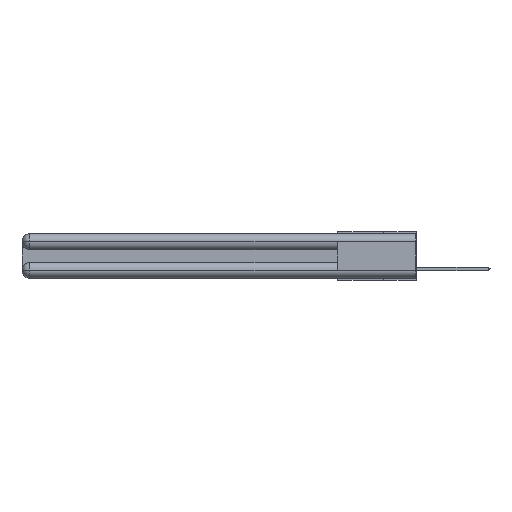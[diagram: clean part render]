
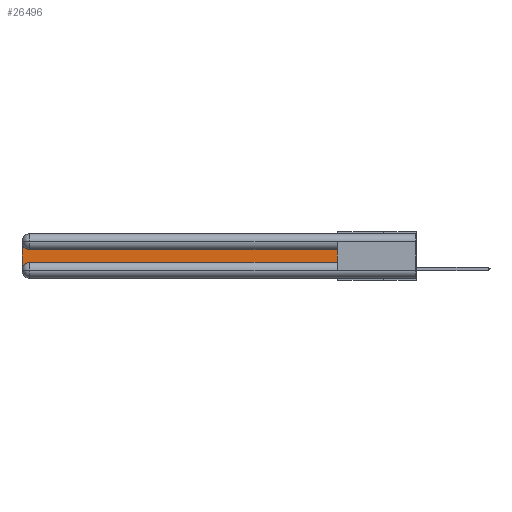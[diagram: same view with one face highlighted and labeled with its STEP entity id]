
A CAD part, left-side view. The second image highlights one B-rep face of the part: STEP entity #26496.
In plain terms, the highlighted planar face has unit normal (-1, 0, 0).
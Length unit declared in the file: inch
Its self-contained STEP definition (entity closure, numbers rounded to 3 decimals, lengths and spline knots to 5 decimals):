
#436 = CARTESIAN_POINT ( 'NONE',  ( 0.075, 2.94, -0.0625 ) ) ;
#612 = ORIENTED_EDGE ( 'NONE', *, *, #9793, .T. ) ;
#1330 = CARTESIAN_POINT ( 'NONE',  ( 0.075, 2.94, -0.2175 ) ) ;
#1367 = CARTESIAN_POINT ( 'NONE',  ( 0.075, 0.6, -0.2175 ) ) ;
#1648 = VERTEX_POINT ( 'NONE', #19882 ) ;
#1867 = DIRECTION ( 'NONE',  ( 0., 0., -1. ) ) ;
#1879 = DIRECTION ( 'NONE',  ( 0., 1., 0. ) ) ;
#2071 = ORIENTED_EDGE ( 'NONE', *, *, #19407, .T. ) ;
#2129 = PLANE ( 'NONE',  #17156 ) ;
#2230 = LINE ( 'NONE', #1367, #27242 ) ;
#2423 = EDGE_LOOP ( 'NONE', ( #29023, #2071, #612, #17621, #30944, #19347 ) ) ;
#3076 = VERTEX_POINT ( 'NONE', #3538 ) ;
#3538 = CARTESIAN_POINT ( 'NONE',  ( 0.075, 2.94, -0.1225 ) ) ;
#5513 = FACE_OUTER_BOUND ( 'NONE', #2423, .T. ) ;
#5653 = DIRECTION ( 'NONE',  ( 1., 0., 0. ) ) ;
#6305 = CARTESIAN_POINT ( 'NONE',  ( 0.075, 3., -0.0625 ) ) ;
#6504 = AXIS2_PLACEMENT_3D ( 'NONE', #436, #5653, #7780 ) ;
#7027 = DIRECTION ( 'NONE',  ( 0., 0., -1. ) ) ;
#7780 = DIRECTION ( 'NONE',  ( 0., 0., -1. ) ) ;
#8475 = VECTOR ( 'NONE', #19235, 39.37008 ) ;
#8689 = VERTEX_POINT ( 'NONE', #6305 ) ;
#9124 = DIRECTION ( 'NONE',  ( 1., 0., 0. ) ) ;
#9793 = EDGE_CURVE ( 'NONE', #8689, #20621, #13392, .T. ) ;
#11976 = CARTESIAN_POINT ( 'NONE',  ( 0.075, 3., -0.1225 ) ) ;
#13082 = CIRCLE ( 'NONE', #6504, 0.06 ) ;
#13392 = LINE ( 'NONE', #21542, #8475 ) ;
#15097 = DIRECTION ( 'NONE',  ( 0., 0., 1. ) ) ;
#15887 = VECTOR ( 'NONE', #15097, 39.37008 ) ;
#16566 = EDGE_CURVE ( 'NONE', #18988, #1648, #20831, .T. ) ;
#17156 = AXIS2_PLACEMENT_3D ( 'NONE', #11976, #9124, #7027 ) ;
#17621 = ORIENTED_EDGE ( 'NONE', *, *, #20976, .T. ) ;
#18319 = DIRECTION ( 'NONE',  ( 0., -1., 0. ) ) ;
#18988 = VERTEX_POINT ( 'NONE', #22869 ) ;
#19011 = CARTESIAN_POINT ( 'NONE',  ( 0.075, 2.94, -0.2775 ) ) ;
#19235 = DIRECTION ( 'NONE',  ( 0., 0., -1. ) ) ;
#19347 = ORIENTED_EDGE ( 'NONE', *, *, #16566, .T. ) ;
#19407 = EDGE_CURVE ( 'NONE', #3076, #8689, #13082, .T. ) ;
#19614 = LINE ( 'NONE', #28260, #20735 ) ;
#19882 = CARTESIAN_POINT ( 'NONE',  ( 0.075, 0.6, -0.1225 ) ) ;
#20621 = VERTEX_POINT ( 'NONE', #22002 ) ;
#20735 = VECTOR ( 'NONE', #1879, 39.37008 ) ;
#20831 = LINE ( 'NONE', #28858, #15887 ) ;
#20976 = EDGE_CURVE ( 'NONE', #20621, #25036, #24670, .T. ) ;
#21542 = CARTESIAN_POINT ( 'NONE',  ( 0.075, 3., -0.2175 ) ) ;
#22002 = CARTESIAN_POINT ( 'NONE',  ( 0.075, 3., -0.2775 ) ) ;
#22869 = CARTESIAN_POINT ( 'NONE',  ( 0.075, 0.6, -0.2175 ) ) ;
#23519 = AXIS2_PLACEMENT_3D ( 'NONE', #19011, #23850, #1867 ) ;
#23850 = DIRECTION ( 'NONE',  ( 1., 0., 0. ) ) ;
#24335 = EDGE_CURVE ( 'NONE', #25036, #18988, #2230, .T. ) ;
#24670 = CIRCLE ( 'NONE', #23519, 0.06 ) ;
#24712 = EDGE_CURVE ( 'NONE', #1648, #3076, #19614, .T. ) ;
#25036 = VERTEX_POINT ( 'NONE', #1330 ) ;
#26496 = ADVANCED_FACE ( 'NONE', ( #5513 ), #2129, .F. ) ;
#27242 = VECTOR ( 'NONE', #18319, 39.37008 ) ;
#28260 = CARTESIAN_POINT ( 'NONE',  ( 0.075, 0.6, -0.1225 ) ) ;
#28858 = CARTESIAN_POINT ( 'NONE',  ( 0.075, 0.6, -0.2175 ) ) ;
#29023 = ORIENTED_EDGE ( 'NONE', *, *, #24712, .T. ) ;
#30944 = ORIENTED_EDGE ( 'NONE', *, *, #24335, .T. ) ;
